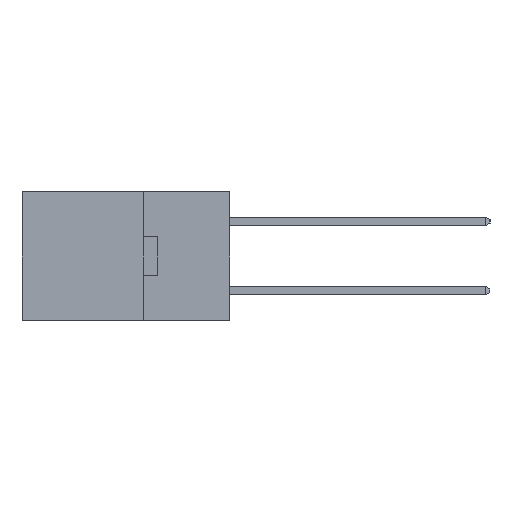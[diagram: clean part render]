
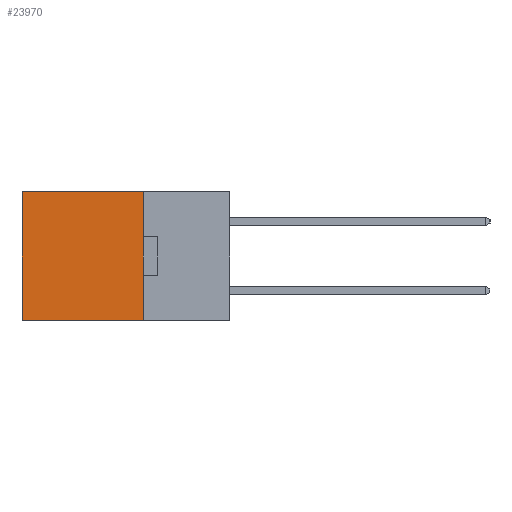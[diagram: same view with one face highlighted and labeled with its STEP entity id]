
A CAD part, left-side view. The second image highlights one B-rep face of the part: STEP entity #23970.
In plain terms, the highlighted planar face has unit normal (-1, 0, 0).
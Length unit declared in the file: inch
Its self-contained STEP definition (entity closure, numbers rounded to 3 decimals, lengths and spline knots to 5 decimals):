
#8 = ORIENTED_EDGE ( 'NONE', *, *, #5571, .F. ) ;
#185 = EDGE_CURVE ( 'NONE', #4539, #3207, #959, .T. ) ;
#258 = ORIENTED_EDGE ( 'NONE', *, *, #4440, .F. ) ;
#532 = DIRECTION ( 'NONE',  ( 0., 0., -1. ) ) ;
#542 = LINE ( 'NONE', #22416, #16689 ) ;
#959 = LINE ( 'NONE', #18170, #23527 ) ;
#3207 = VERTEX_POINT ( 'NONE', #25580 ) ;
#4440 = EDGE_CURVE ( 'NONE', #24524, #10955, #27230, .T. ) ;
#4539 = VERTEX_POINT ( 'NONE', #12394 ) ;
#5395 = CARTESIAN_POINT ( 'NONE',  ( 0.2615, 0.6, -0.37 ) ) ;
#5571 = EDGE_CURVE ( 'NONE', #4539, #24524, #542, .T. ) ;
#6433 = DIRECTION ( 'NONE',  ( 0., 0., -1. ) ) ;
#7786 = EDGE_LOOP ( 'NONE', ( #17623, #258, #8, #24891 ) ) ;
#10229 = VECTOR ( 'NONE', #22850, 39.37008 ) ;
#10955 = VERTEX_POINT ( 'NONE', #18755 ) ;
#12394 = CARTESIAN_POINT ( 'NONE',  ( 0.2615, 0.25, 0. ) ) ;
#14229 = EDGE_CURVE ( 'NONE', #3207, #10955, #16066, .T. ) ;
#14314 = CARTESIAN_POINT ( 'NONE',  ( 0.2615, 0.25, -0.37 ) ) ;
#15048 = VECTOR ( 'NONE', #27289, 39.37008 ) ;
#15173 = PLANE ( 'NONE',  #26546 ) ;
#16066 = LINE ( 'NONE', #5395, #10229 ) ;
#16689 = VECTOR ( 'NONE', #532, 39.37008 ) ;
#17359 = CARTESIAN_POINT ( 'NONE',  ( 0.2615, 0.25, -0.37 ) ) ;
#17623 = ORIENTED_EDGE ( 'NONE', *, *, #14229, .T. ) ;
#17759 = DIRECTION ( 'NONE',  ( 0., 1., 0. ) ) ;
#18170 = CARTESIAN_POINT ( 'NONE',  ( 0.2615, 0.25, 0. ) ) ;
#18755 = CARTESIAN_POINT ( 'NONE',  ( 0.2615, 0.6, -0.37 ) ) ;
#19104 = FACE_OUTER_BOUND ( 'NONE', #7786, .T. ) ;
#19542 = DIRECTION ( 'NONE',  ( 1., 0., 0. ) ) ;
#22416 = CARTESIAN_POINT ( 'NONE',  ( 0.2615, 0.25, -0.37 ) ) ;
#22850 = DIRECTION ( 'NONE',  ( 0., 0., -1. ) ) ;
#23527 = VECTOR ( 'NONE', #17759, 39.37008 ) ;
#23970 = ADVANCED_FACE ( 'NONE', ( #19104 ), #15173, .F. ) ;
#24524 = VERTEX_POINT ( 'NONE', #25471 ) ;
#24891 = ORIENTED_EDGE ( 'NONE', *, *, #185, .T. ) ;
#25471 = CARTESIAN_POINT ( 'NONE',  ( 0.2615, 0.25, -0.37 ) ) ;
#25580 = CARTESIAN_POINT ( 'NONE',  ( 0.2615, 0.6, 0. ) ) ;
#26546 = AXIS2_PLACEMENT_3D ( 'NONE', #17359, #19542, #6433 ) ;
#27230 = LINE ( 'NONE', #14314, #15048 ) ;
#27289 = DIRECTION ( 'NONE',  ( 0., 1., 0. ) ) ;
